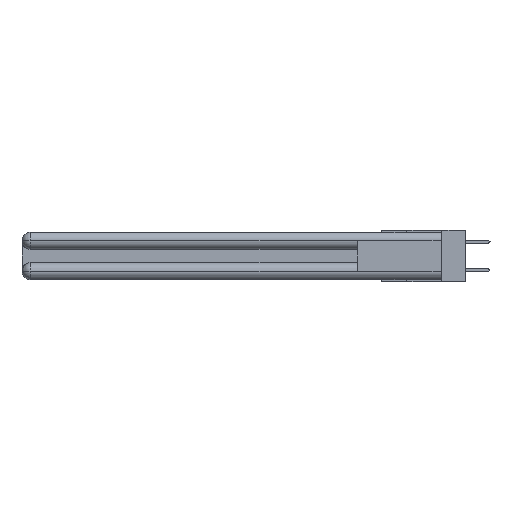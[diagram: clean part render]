
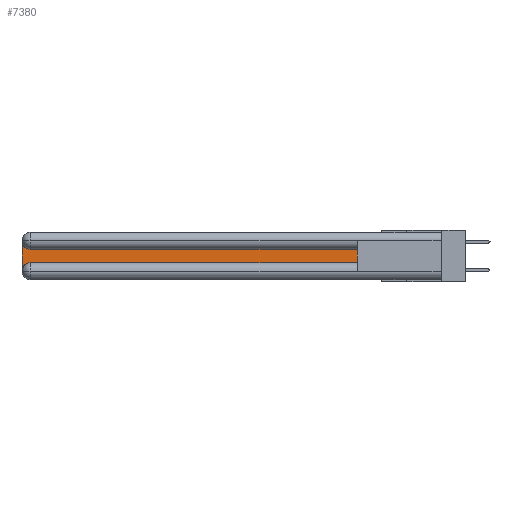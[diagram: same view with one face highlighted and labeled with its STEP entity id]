
A CAD part, left-side view. The second image highlights one B-rep face of the part: STEP entity #7380.
In plain terms, the highlighted planar face has unit normal (-1, 0, 0).
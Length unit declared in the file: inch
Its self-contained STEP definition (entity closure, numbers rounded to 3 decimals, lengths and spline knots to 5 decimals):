
#91 = CIRCLE ( 'NONE', #8290, 0.06 ) ;
#243 = VECTOR ( 'NONE', #27373, 39.37008 ) ;
#1087 = AXIS2_PLACEMENT_3D ( 'NONE', #13795, #32569, #3218 ) ;
#1249 = CARTESIAN_POINT ( 'NONE',  ( 0.075, 3., -0.1225 ) ) ;
#1948 = AXIS2_PLACEMENT_3D ( 'NONE', #1249, #3823, #25374 ) ;
#3114 = CARTESIAN_POINT ( 'NONE',  ( 0.075, 3., -0.2175 ) ) ;
#3192 = ORIENTED_EDGE ( 'NONE', *, *, #16177, .T. ) ;
#3218 = DIRECTION ( 'NONE',  ( 0., 0., -1. ) ) ;
#3418 = VERTEX_POINT ( 'NONE', #13766 ) ;
#3823 = DIRECTION ( 'NONE',  ( 1., 0., 0. ) ) ;
#6129 = VERTEX_POINT ( 'NONE', #23772 ) ;
#6426 = CARTESIAN_POINT ( 'NONE',  ( 0.075, 3., -0.0625 ) ) ;
#7132 = LINE ( 'NONE', #34673, #22323 ) ;
#7380 = ADVANCED_FACE ( 'NONE', ( #7792 ), #25499, .F. ) ;
#7792 = FACE_OUTER_BOUND ( 'NONE', #31616, .T. ) ;
#8290 = AXIS2_PLACEMENT_3D ( 'NONE', #15270, #11428, #21756 ) ;
#9097 = EDGE_CURVE ( 'NONE', #15937, #32553, #91, .T. ) ;
#9217 = DIRECTION ( 'NONE',  ( 0., 1., 0. ) ) ;
#10470 = ORIENTED_EDGE ( 'NONE', *, *, #19345, .T. ) ;
#10592 = DIRECTION ( 'NONE',  ( 0., 0., 1. ) ) ;
#11428 = DIRECTION ( 'NONE',  ( 1., 0., 0. ) ) ;
#11573 = CARTESIAN_POINT ( 'NONE',  ( 0.075, 0.6, -0.2175 ) ) ;
#12906 = EDGE_CURVE ( 'NONE', #6129, #3418, #21431, .T. ) ;
#13766 = CARTESIAN_POINT ( 'NONE',  ( 0.075, 0.6, -0.2175 ) ) ;
#13795 = CARTESIAN_POINT ( 'NONE',  ( 0.075, 2.94, -0.2775 ) ) ;
#15270 = CARTESIAN_POINT ( 'NONE',  ( 0.075, 2.94, -0.0625 ) ) ;
#15937 = VERTEX_POINT ( 'NONE', #24883 ) ;
#16177 = EDGE_CURVE ( 'NONE', #24539, #15937, #33263, .T. ) ;
#16497 = VECTOR ( 'NONE', #9217, 39.37008 ) ;
#17159 = VECTOR ( 'NONE', #27721, 39.37008 ) ;
#19288 = CARTESIAN_POINT ( 'NONE',  ( 0.075, 0.6, -0.1225 ) ) ;
#19345 = EDGE_CURVE ( 'NONE', #3418, #24539, #7132, .T. ) ;
#21431 = LINE ( 'NONE', #11573, #17159 ) ;
#21756 = DIRECTION ( 'NONE',  ( 0., 0., -1. ) ) ;
#21794 = EDGE_CURVE ( 'NONE', #32553, #22588, #33819, .T. ) ;
#21826 = CARTESIAN_POINT ( 'NONE',  ( 0.075, 3., -0.2775 ) ) ;
#22189 = ORIENTED_EDGE ( 'NONE', *, *, #33851, .T. ) ;
#22323 = VECTOR ( 'NONE', #10592, 39.37008 ) ;
#22588 = VERTEX_POINT ( 'NONE', #21826 ) ;
#23772 = CARTESIAN_POINT ( 'NONE',  ( 0.075, 2.94, -0.2175 ) ) ;
#24216 = CIRCLE ( 'NONE', #1087, 0.06 ) ;
#24539 = VERTEX_POINT ( 'NONE', #19288 ) ;
#24883 = CARTESIAN_POINT ( 'NONE',  ( 0.075, 2.94, -0.1225 ) ) ;
#25025 = CARTESIAN_POINT ( 'NONE',  ( 0.075, 0.6, -0.1225 ) ) ;
#25374 = DIRECTION ( 'NONE',  ( 0., 0., -1. ) ) ;
#25499 = PLANE ( 'NONE',  #1948 ) ;
#27373 = DIRECTION ( 'NONE',  ( 0., 0., -1. ) ) ;
#27721 = DIRECTION ( 'NONE',  ( 0., -1., 0. ) ) ;
#28410 = ORIENTED_EDGE ( 'NONE', *, *, #21794, .T. ) ;
#29712 = ORIENTED_EDGE ( 'NONE', *, *, #9097, .T. ) ;
#31616 = EDGE_LOOP ( 'NONE', ( #3192, #29712, #28410, #22189, #33412, #10470 ) ) ;
#32553 = VERTEX_POINT ( 'NONE', #6426 ) ;
#32569 = DIRECTION ( 'NONE',  ( 1., 0., 0. ) ) ;
#33263 = LINE ( 'NONE', #25025, #16497 ) ;
#33412 = ORIENTED_EDGE ( 'NONE', *, *, #12906, .T. ) ;
#33819 = LINE ( 'NONE', #3114, #243 ) ;
#33851 = EDGE_CURVE ( 'NONE', #22588, #6129, #24216, .T. ) ;
#34673 = CARTESIAN_POINT ( 'NONE',  ( 0.075, 0.6, -0.2175 ) ) ;
